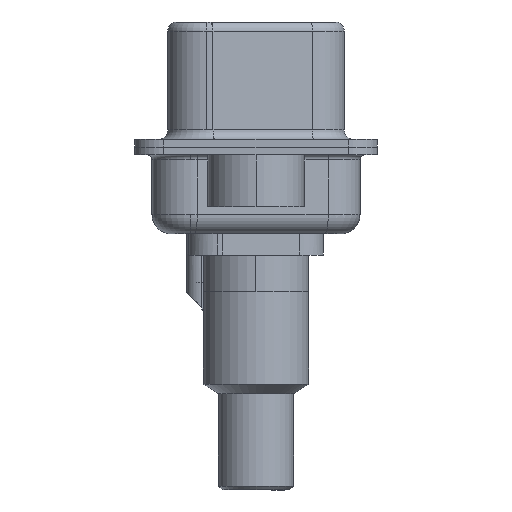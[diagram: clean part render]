
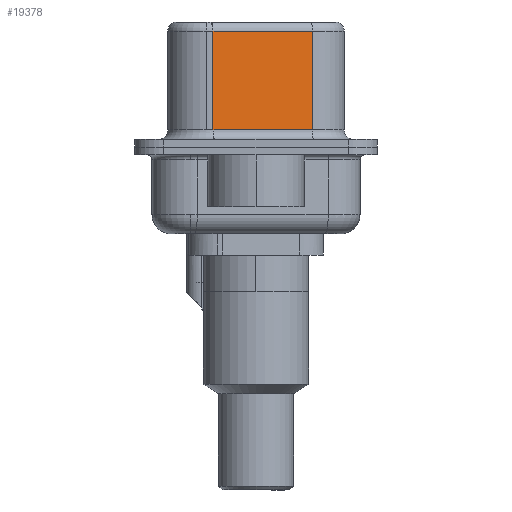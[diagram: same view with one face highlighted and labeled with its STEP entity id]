
A CAD part, left-side view. The second image highlights one B-rep face of the part: STEP entity #19378.
In plain terms, the highlighted planar face has unit normal (-0.985, -0.174, 0).
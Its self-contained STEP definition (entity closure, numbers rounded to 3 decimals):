
#342 = ORIENTED_EDGE ( 'NONE', *, *, #17501, .T. ) ;
#1371 = DIRECTION ( 'NONE',  ( 0., 0., -1. ) ) ;
#2846 = FACE_OUTER_BOUND ( 'NONE', #23094, .T. ) ;
#2992 = PLANE ( 'NONE',  #19468 ) ;
#3063 = DIRECTION ( 'NONE',  ( -0.174, 0.985, 0. ) ) ;
#3580 = VECTOR ( 'NONE', #11475, 1000. ) ;
#4175 = ORIENTED_EDGE ( 'NONE', *, *, #22489, .F. ) ;
#5244 = LINE ( 'NONE', #23345, #19733 ) ;
#6574 = CARTESIAN_POINT ( 'NONE',  ( 3.67, 2.233, 0.9 ) ) ;
#6894 = CARTESIAN_POINT ( 'NONE',  ( 4.58, -2.927, 0.9 ) ) ;
#7416 = CARTESIAN_POINT ( 'NONE',  ( 3.67, 2.233, 6.02 ) ) ;
#7488 = VECTOR ( 'NONE', #10405, 1000. ) ;
#9265 = VERTEX_POINT ( 'NONE', #12649 ) ;
#9833 = VERTEX_POINT ( 'NONE', #6894 ) ;
#10405 = DIRECTION ( 'NONE',  ( 0., 0., -1. ) ) ;
#10445 = DIRECTION ( 'NONE',  ( 0.174, -0.985, 0. ) ) ;
#11475 = DIRECTION ( 'NONE',  ( -0.174, 0.985, 0. ) ) ;
#11664 = LINE ( 'NONE', #15942, #7488 ) ;
#12649 = CARTESIAN_POINT ( 'NONE',  ( 4.58, -2.927, 6.02 ) ) ;
#13647 = VERTEX_POINT ( 'NONE', #7416 ) ;
#13910 = DIRECTION ( 'NONE',  ( 0.985, 0.174, 0. ) ) ;
#14058 = VECTOR ( 'NONE', #1371, 1000. ) ;
#15229 = ORIENTED_EDGE ( 'NONE', *, *, #23654, .T. ) ;
#15942 = CARTESIAN_POINT ( 'NONE',  ( 3.67, 2.233, 6.52 ) ) ;
#16399 = ORIENTED_EDGE ( 'NONE', *, *, #22853, .T. ) ;
#17376 = VERTEX_POINT ( 'NONE', #6574 ) ;
#17501 = EDGE_CURVE ( 'NONE', #17376, #9833, #5244, .T. ) ;
#18932 = LINE ( 'NONE', #23276, #14058 ) ;
#19378 = ADVANCED_FACE ( 'NONE', ( #2846 ), #2992, .F. ) ;
#19468 = AXIS2_PLACEMENT_3D ( 'NONE', #21275, #13910, #3063 ) ;
#19733 = VECTOR ( 'NONE', #10445, 1000. ) ;
#21275 = CARTESIAN_POINT ( 'NONE',  ( 4.58, -2.927, 6.52 ) ) ;
#21277 = LINE ( 'NONE', #22555, #3580 ) ;
#22489 = EDGE_CURVE ( 'NONE', #9265, #9833, #18932, .T. ) ;
#22555 = CARTESIAN_POINT ( 'NONE',  ( 4.58, -2.927, 6.02 ) ) ;
#22853 = EDGE_CURVE ( 'NONE', #9265, #13647, #21277, .T. ) ;
#23094 = EDGE_LOOP ( 'NONE', ( #4175, #16399, #15229, #342 ) ) ;
#23276 = CARTESIAN_POINT ( 'NONE',  ( 4.58, -2.927, 6.52 ) ) ;
#23345 = CARTESIAN_POINT ( 'NONE',  ( 4.58, -2.927, 0.9 ) ) ;
#23654 = EDGE_CURVE ( 'NONE', #13647, #17376, #11664, .T. ) ;
